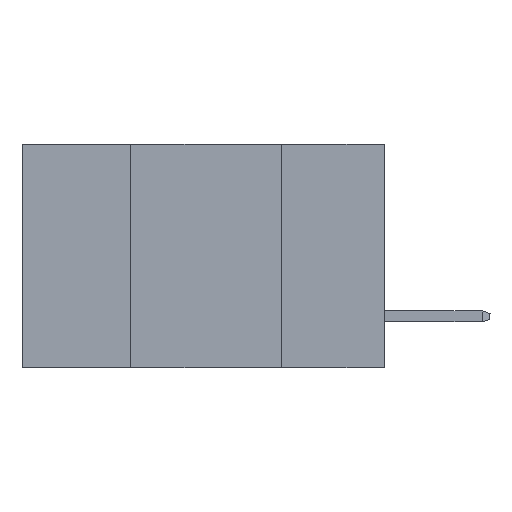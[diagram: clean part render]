
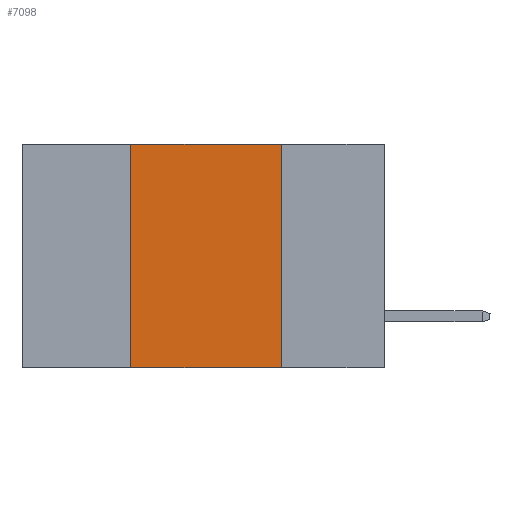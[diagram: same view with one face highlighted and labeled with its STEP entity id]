
A CAD part, left-side view. The second image highlights one B-rep face of the part: STEP entity #7098.
In plain terms, the highlighted planar face has unit normal (-1, 0, 0).
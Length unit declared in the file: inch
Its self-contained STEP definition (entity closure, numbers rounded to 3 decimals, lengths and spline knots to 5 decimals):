
#302 = EDGE_LOOP ( 'NONE', ( #1583, #13963, #7307, #6851 ) ) ;
#444 = DIRECTION ( 'NONE',  ( 0., -1., 0. ) ) ;
#784 = CARTESIAN_POINT ( 'NONE',  ( 0., 0.6, 0. ) ) ;
#1583 = ORIENTED_EDGE ( 'NONE', *, *, #14164, .F. ) ;
#1824 = LINE ( 'NONE', #7295, #13856 ) ;
#2846 = CARTESIAN_POINT ( 'NONE',  ( 0., 0.6, -0.37 ) ) ;
#2895 = CARTESIAN_POINT ( 'NONE',  ( 0., 0.17, -0.37 ) ) ;
#3122 = EDGE_CURVE ( 'NONE', #6166, #14420, #1824, .T. ) ;
#3251 = PLANE ( 'NONE',  #13248 ) ;
#3622 = CARTESIAN_POINT ( 'NONE',  ( 0., 0.42, 0. ) ) ;
#4001 = VECTOR ( 'NONE', #11118, 39.37008 ) ;
#5057 = CARTESIAN_POINT ( 'NONE',  ( 0., 0.17, 0. ) ) ;
#5360 = DIRECTION ( 'NONE',  ( 0., 0., -1. ) ) ;
#6166 = VERTEX_POINT ( 'NONE', #7565 ) ;
#6225 = LINE ( 'NONE', #8313, #12111 ) ;
#6851 = ORIENTED_EDGE ( 'NONE', *, *, #10857, .T. ) ;
#7098 = ADVANCED_FACE ( 'NONE', ( #12177 ), #3251, .F. ) ;
#7295 = CARTESIAN_POINT ( 'NONE',  ( 0., 0.42, -0.37 ) ) ;
#7307 = ORIENTED_EDGE ( 'NONE', *, *, #3122, .F. ) ;
#7420 = DIRECTION ( 'NONE',  ( 0., -1., 0. ) ) ;
#7565 = CARTESIAN_POINT ( 'NONE',  ( 0., 0.42, -0.37 ) ) ;
#7598 = LINE ( 'NONE', #2895, #4001 ) ;
#7817 = DIRECTION ( 'NONE',  ( 1., 0., 0. ) ) ;
#8313 = CARTESIAN_POINT ( 'NONE',  ( 0., 0.6, 0. ) ) ;
#9683 = DIRECTION ( 'NONE',  ( 0., 0., 1. ) ) ;
#9926 = VERTEX_POINT ( 'NONE', #5057 ) ;
#9939 = LINE ( 'NONE', #2846, #11504 ) ;
#10857 = EDGE_CURVE ( 'NONE', #6166, #14478, #9939, .T. ) ;
#11118 = DIRECTION ( 'NONE',  ( 0., 0., -1. ) ) ;
#11303 = CARTESIAN_POINT ( 'NONE',  ( 0., 0.17, -0.37 ) ) ;
#11504 = VECTOR ( 'NONE', #7420, 39.37008 ) ;
#12111 = VECTOR ( 'NONE', #444, 39.37008 ) ;
#12121 = EDGE_CURVE ( 'NONE', #14420, #9926, #6225, .T. ) ;
#12177 = FACE_OUTER_BOUND ( 'NONE', #302, .T. ) ;
#13248 = AXIS2_PLACEMENT_3D ( 'NONE', #784, #7817, #5360 ) ;
#13856 = VECTOR ( 'NONE', #9683, 39.37008 ) ;
#13963 = ORIENTED_EDGE ( 'NONE', *, *, #12121, .F. ) ;
#14164 = EDGE_CURVE ( 'NONE', #9926, #14478, #7598, .T. ) ;
#14420 = VERTEX_POINT ( 'NONE', #3622 ) ;
#14478 = VERTEX_POINT ( 'NONE', #11303 ) ;
